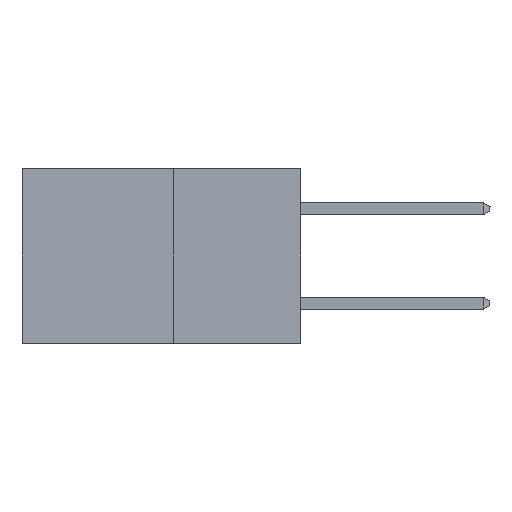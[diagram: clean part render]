
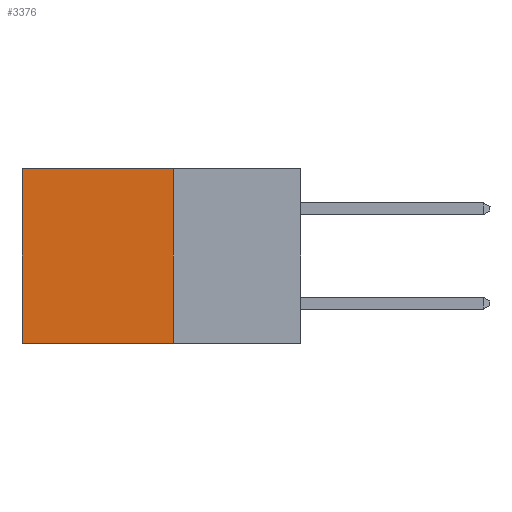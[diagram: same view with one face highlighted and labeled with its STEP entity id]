
A CAD part, left-side view. The second image highlights one B-rep face of the part: STEP entity #3376.
In plain terms, the highlighted planar face has unit normal (-1, 0, 0).
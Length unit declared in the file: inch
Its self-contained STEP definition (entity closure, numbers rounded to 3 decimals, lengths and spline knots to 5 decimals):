
#27 = DIRECTION ( 'NONE',  ( 0., 0., -1. ) ) ;
#102 = DIRECTION ( 'NONE',  ( 1., 0., 0. ) ) ;
#332 = VERTEX_POINT ( 'NONE', #1568 ) ;
#615 = LINE ( 'NONE', #7400, #4960 ) ;
#1568 = CARTESIAN_POINT ( 'NONE',  ( 0.277, 0.27, 0. ) ) ;
#1601 = EDGE_CURVE ( 'NONE', #7635, #7398, #615, .T. ) ;
#1752 = ORIENTED_EDGE ( 'NONE', *, *, #5883, .F. ) ;
#2008 = CARTESIAN_POINT ( 'NONE',  ( 0.277, 0.59, 0. ) ) ;
#2079 = DIRECTION ( 'NONE',  ( 0., 1., 0. ) ) ;
#2214 = EDGE_CURVE ( 'NONE', #332, #10935, #3776, .T. ) ;
#2391 = VECTOR ( 'NONE', #7638, 39.37008 ) ;
#3376 = ADVANCED_FACE ( 'NONE', ( #10470 ), #4480, .F. ) ;
#3497 = VECTOR ( 'NONE', #2079, 39.37008 ) ;
#3544 = VECTOR ( 'NONE', #9471, 39.37008 ) ;
#3630 = CARTESIAN_POINT ( 'NONE',  ( 0.277, 0.27, -0.37 ) ) ;
#3776 = LINE ( 'NONE', #7600, #3497 ) ;
#4360 = AXIS2_PLACEMENT_3D ( 'NONE', #4719, #102, #27 ) ;
#4480 = PLANE ( 'NONE',  #4360 ) ;
#4558 = CARTESIAN_POINT ( 'NONE',  ( 0.277, 0.59, -0.37 ) ) ;
#4719 = CARTESIAN_POINT ( 'NONE',  ( 0.277, 0.27, -0.37 ) ) ;
#4960 = VECTOR ( 'NONE', #7357, 39.37008 ) ;
#5488 = EDGE_LOOP ( 'NONE', ( #10213, #10506, #1752, #9185 ) ) ;
#5883 = EDGE_CURVE ( 'NONE', #332, #7635, #6035, .T. ) ;
#6017 = EDGE_CURVE ( 'NONE', #10935, #7398, #11793, .T. ) ;
#6035 = LINE ( 'NONE', #9864, #3544 ) ;
#7357 = DIRECTION ( 'NONE',  ( 0., 1., 0. ) ) ;
#7398 = VERTEX_POINT ( 'NONE', #4558 ) ;
#7400 = CARTESIAN_POINT ( 'NONE',  ( 0.277, 0.27, -0.37 ) ) ;
#7600 = CARTESIAN_POINT ( 'NONE',  ( 0.277, 0.27, 0. ) ) ;
#7635 = VERTEX_POINT ( 'NONE', #3630 ) ;
#7638 = DIRECTION ( 'NONE',  ( 0., 0., -1. ) ) ;
#7648 = CARTESIAN_POINT ( 'NONE',  ( 0.277, 0.59, -0.37 ) ) ;
#9185 = ORIENTED_EDGE ( 'NONE', *, *, #2214, .T. ) ;
#9471 = DIRECTION ( 'NONE',  ( 0., 0., -1. ) ) ;
#9864 = CARTESIAN_POINT ( 'NONE',  ( 0.277, 0.27, -0.37 ) ) ;
#10213 = ORIENTED_EDGE ( 'NONE', *, *, #6017, .T. ) ;
#10470 = FACE_OUTER_BOUND ( 'NONE', #5488, .T. ) ;
#10506 = ORIENTED_EDGE ( 'NONE', *, *, #1601, .F. ) ;
#10935 = VERTEX_POINT ( 'NONE', #2008 ) ;
#11793 = LINE ( 'NONE', #7648, #2391 ) ;
